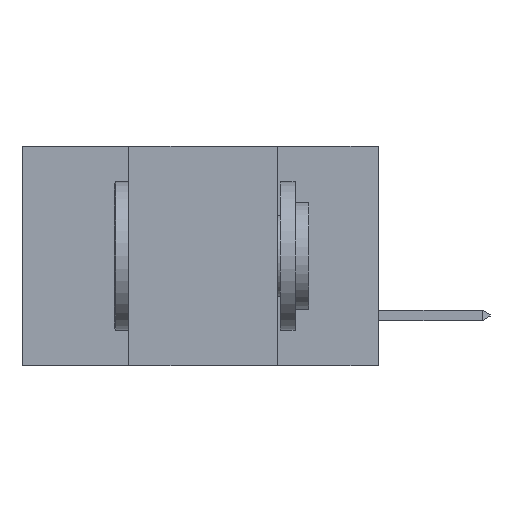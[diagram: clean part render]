
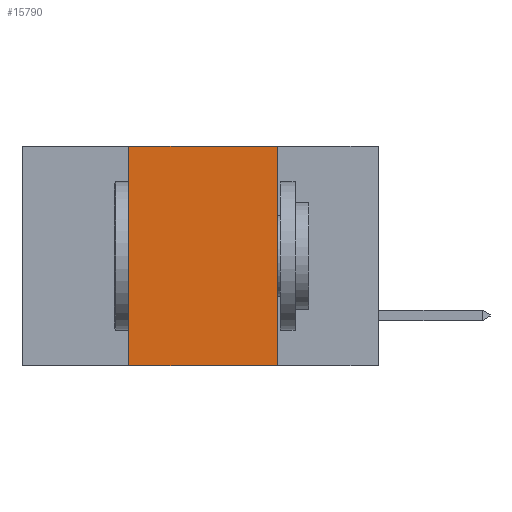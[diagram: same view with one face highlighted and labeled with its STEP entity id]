
A CAD part, left-side view. The second image highlights one B-rep face of the part: STEP entity #15790.
In plain terms, the highlighted planar face has unit normal (-1, 0, 0).
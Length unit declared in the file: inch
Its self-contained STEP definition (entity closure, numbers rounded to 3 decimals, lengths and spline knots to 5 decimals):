
#974 = ORIENTED_EDGE ( 'NONE', *, *, #3598, .F. ) ;
#1062 = CARTESIAN_POINT ( 'NONE',  ( 0., 0.42, 0. ) ) ;
#1102 = ORIENTED_EDGE ( 'NONE', *, *, #9900, .F. ) ;
#1117 = ORIENTED_EDGE ( 'NONE', *, *, #5373, .F. ) ;
#1197 = ORIENTED_EDGE ( 'NONE', *, *, #6209, .T. ) ;
#1590 = CARTESIAN_POINT ( 'NONE',  ( 0., 0.6, -0.37 ) ) ;
#1640 = DIRECTION ( 'NONE',  ( 0., -1., 0. ) ) ;
#1676 = VECTOR ( 'NONE', #9510, 39.37008 ) ;
#2820 = DIRECTION ( 'NONE',  ( 1., 0., 0. ) ) ;
#3598 = EDGE_CURVE ( 'NONE', #6292, #4337, #5116, .T. ) ;
#3683 = FACE_OUTER_BOUND ( 'NONE', #5468, .T. ) ;
#4004 = CARTESIAN_POINT ( 'NONE',  ( 0., 0.42, 0. ) ) ;
#4337 = VERTEX_POINT ( 'NONE', #8926 ) ;
#5116 = LINE ( 'NONE', #9555, #1676 ) ;
#5200 = CARTESIAN_POINT ( 'NONE',  ( 0., 0.6, 0. ) ) ;
#5244 = AXIS2_PLACEMENT_3D ( 'NONE', #10400, #2820, #11603 ) ;
#5373 = EDGE_CURVE ( 'NONE', #7868, #6496, #12617, .T. ) ;
#5468 = EDGE_LOOP ( 'NONE', ( #974, #1102, #1117, #1197 ) ) ;
#6209 = EDGE_CURVE ( 'NONE', #7868, #4337, #16172, .T. ) ;
#6292 = VERTEX_POINT ( 'NONE', #15005 ) ;
#6433 = VECTOR ( 'NONE', #1640, 39.37008 ) ;
#6463 = DIRECTION ( 'NONE',  ( 0., -1., 0. ) ) ;
#6496 = VERTEX_POINT ( 'NONE', #4004 ) ;
#6621 = PLANE ( 'NONE',  #5244 ) ;
#7868 = VERTEX_POINT ( 'NONE', #12276 ) ;
#8128 = VECTOR ( 'NONE', #6463, 39.37008 ) ;
#8926 = CARTESIAN_POINT ( 'NONE',  ( 0., 0.17, -0.37 ) ) ;
#9413 = VECTOR ( 'NONE', #11002, 39.37008 ) ;
#9510 = DIRECTION ( 'NONE',  ( 0., 0., -1. ) ) ;
#9555 = CARTESIAN_POINT ( 'NONE',  ( 0., 0.17, 0. ) ) ;
#9900 = EDGE_CURVE ( 'NONE', #6496, #6292, #14978, .T. ) ;
#10400 = CARTESIAN_POINT ( 'NONE',  ( 0., 0.6, 0. ) ) ;
#11002 = DIRECTION ( 'NONE',  ( 0., 0., 1. ) ) ;
#11603 = DIRECTION ( 'NONE',  ( 0., 0., -1. ) ) ;
#12276 = CARTESIAN_POINT ( 'NONE',  ( 0., 0.42, -0.37 ) ) ;
#12617 = LINE ( 'NONE', #1062, #9413 ) ;
#14978 = LINE ( 'NONE', #5200, #8128 ) ;
#15005 = CARTESIAN_POINT ( 'NONE',  ( 0., 0.17, 0. ) ) ;
#15790 = ADVANCED_FACE ( 'NONE', ( #3683 ), #6621, .F. ) ;
#16172 = LINE ( 'NONE', #1590, #6433 ) ;
